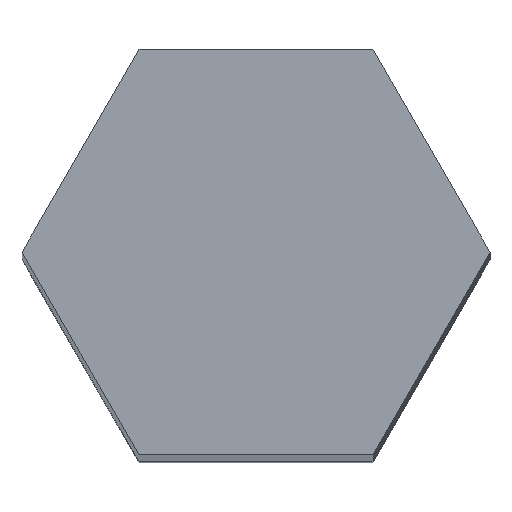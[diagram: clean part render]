
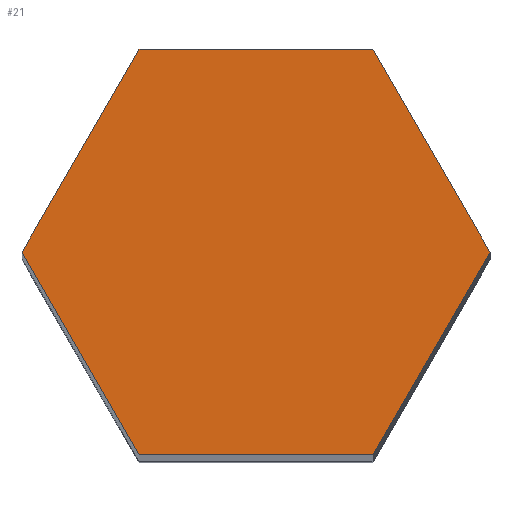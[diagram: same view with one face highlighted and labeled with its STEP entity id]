
A CAD part, top view. The second image highlights one B-rep face of the part: STEP entity #21.
In plain terms, the highlighted planar face has unit normal (0, 0, 1).
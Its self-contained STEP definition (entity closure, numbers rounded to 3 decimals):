
#20 = EDGE_CURVE ( 'NONE', #51, #489, #417, .T. ) ;
#21 = ADVANCED_FACE ( 'NONE', ( #457 ), #455, .T. ) ;
#29 = CARTESIAN_POINT ( 'NONE',  ( 3.666, -6.35, 142. ) ) ;
#36 = VECTOR ( 'NONE', #91, 1000. ) ;
#37 = DIRECTION ( 'NONE',  ( 0., 0., 1. ) ) ;
#40 = CARTESIAN_POINT ( 'NONE',  ( -3.666, -6.35, 142. ) ) ;
#43 = LINE ( 'NONE', #48, #36 ) ;
#44 = VECTOR ( 'NONE', #193, 1000. ) ;
#48 = CARTESIAN_POINT ( 'NONE',  ( 7.332, 0., 142. ) ) ;
#51 = VERTEX_POINT ( 'NONE', #335 ) ;
#91 = DIRECTION ( 'NONE',  ( -0.5, 0.866, 0. ) ) ;
#106 = LINE ( 'NONE', #363, #330 ) ;
#112 = LINE ( 'NONE', #197, #44 ) ;
#123 = VECTOR ( 'NONE', #474, 1000. ) ;
#182 = LINE ( 'NONE', #423, #530 ) ;
#190 = ORIENTED_EDGE ( 'NONE', *, *, #412, .T. ) ;
#193 = DIRECTION ( 'NONE',  ( -1., 0., 0. ) ) ;
#197 = CARTESIAN_POINT ( 'NONE',  ( 3.666, 6.35, 142. ) ) ;
#198 = VERTEX_POINT ( 'NONE', #398 ) ;
#200 = AXIS2_PLACEMENT_3D ( 'NONE', #415, #37, #207 ) ;
#202 = EDGE_LOOP ( 'NONE', ( #278, #519, #190, #448, #409, #312 ) ) ;
#207 = DIRECTION ( 'NONE',  ( 1., 0., 0. ) ) ;
#208 = EDGE_CURVE ( 'NONE', #378, #198, #43, .T. ) ;
#250 = DIRECTION ( 'NONE',  ( -0.5, -0.866, 0. ) ) ;
#278 = ORIENTED_EDGE ( 'NONE', *, *, #377, .T. ) ;
#283 = EDGE_CURVE ( 'NONE', #198, #51, #112, .T. ) ;
#290 = CARTESIAN_POINT ( 'NONE',  ( -3.666, 6.35, 142. ) ) ;
#312 = ORIENTED_EDGE ( 'NONE', *, *, #20, .T. ) ;
#317 = EDGE_CURVE ( 'NONE', #523, #326, #106, .T. ) ;
#326 = VERTEX_POINT ( 'NONE', #29 ) ;
#330 = VECTOR ( 'NONE', #442, 1000. ) ;
#335 = CARTESIAN_POINT ( 'NONE',  ( -3.666, 6.35, 142. ) ) ;
#363 = CARTESIAN_POINT ( 'NONE',  ( -3.666, -6.35, 142. ) ) ;
#377 = EDGE_CURVE ( 'NONE', #489, #523, #379, .T. ) ;
#378 = VERTEX_POINT ( 'NONE', #513 ) ;
#379 = LINE ( 'NONE', #429, #123 ) ;
#398 = CARTESIAN_POINT ( 'NONE',  ( 3.666, 6.35, 142. ) ) ;
#409 = ORIENTED_EDGE ( 'NONE', *, *, #283, .T. ) ;
#412 = EDGE_CURVE ( 'NONE', #326, #378, #182, .T. ) ;
#415 = CARTESIAN_POINT ( 'NONE',  ( 0., 0., 142. ) ) ;
#417 = LINE ( 'NONE', #290, #537 ) ;
#423 = CARTESIAN_POINT ( 'NONE',  ( 3.666, -6.35, 142. ) ) ;
#429 = CARTESIAN_POINT ( 'NONE',  ( -7.332, 0., 142. ) ) ;
#442 = DIRECTION ( 'NONE',  ( 1., 0., 0. ) ) ;
#448 = ORIENTED_EDGE ( 'NONE', *, *, #208, .T. ) ;
#455 = PLANE ( 'NONE',  #200 ) ;
#457 = FACE_OUTER_BOUND ( 'NONE', #202, .T. ) ;
#460 = DIRECTION ( 'NONE',  ( 0.5, 0.866, 0. ) ) ;
#468 = CARTESIAN_POINT ( 'NONE',  ( -7.332, 0., 142. ) ) ;
#474 = DIRECTION ( 'NONE',  ( 0.5, -0.866, 0. ) ) ;
#489 = VERTEX_POINT ( 'NONE', #468 ) ;
#513 = CARTESIAN_POINT ( 'NONE',  ( 7.332, 0., 142. ) ) ;
#519 = ORIENTED_EDGE ( 'NONE', *, *, #317, .T. ) ;
#523 = VERTEX_POINT ( 'NONE', #40 ) ;
#530 = VECTOR ( 'NONE', #460, 1000. ) ;
#537 = VECTOR ( 'NONE', #250, 1000. ) ;
